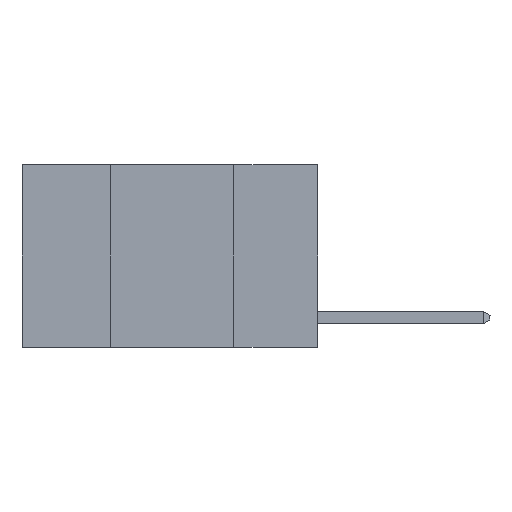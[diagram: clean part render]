
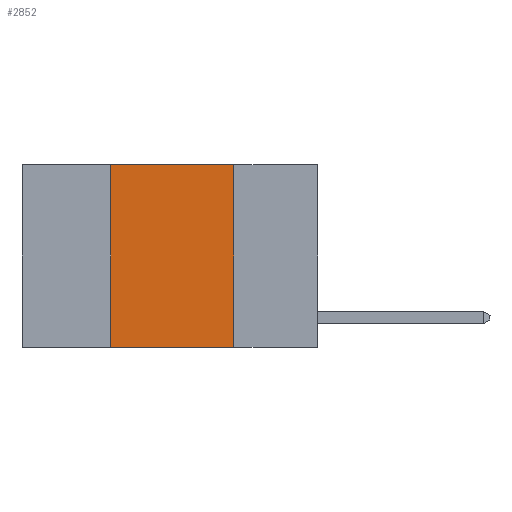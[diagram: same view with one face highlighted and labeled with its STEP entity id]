
A CAD part, left-side view. The second image highlights one B-rep face of the part: STEP entity #2852.
In plain terms, the highlighted planar face has unit normal (-1, 0, 0).
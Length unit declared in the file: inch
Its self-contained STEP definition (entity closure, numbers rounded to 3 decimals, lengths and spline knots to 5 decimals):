
#389 = CARTESIAN_POINT ( 'NONE',  ( 0., 0.42, 0. ) ) ;
#398 = DIRECTION ( 'NONE',  ( 0., -1., 0. ) ) ;
#1390 = VERTEX_POINT ( 'NONE', #5382 ) ;
#2214 = VERTEX_POINT ( 'NONE', #13376 ) ;
#2626 = EDGE_CURVE ( 'NONE', #2214, #1390, #2930, .T. ) ;
#2852 = ADVANCED_FACE ( 'NONE', ( #9622 ), #25885, .F. ) ;
#2920 = DIRECTION ( 'NONE',  ( 0., -1., 0. ) ) ;
#2930 = LINE ( 'NONE', #18603, #17862 ) ;
#4435 = EDGE_CURVE ( 'NONE', #23486, #2214, #18718, .T. ) ;
#4903 = CARTESIAN_POINT ( 'NONE',  ( 0., 0.17, -0.37 ) ) ;
#5269 = ORIENTED_EDGE ( 'NONE', *, *, #13806, .F. ) ;
#5382 = CARTESIAN_POINT ( 'NONE',  ( 0., 0.17, 0. ) ) ;
#5502 = CARTESIAN_POINT ( 'NONE',  ( 0., 0.17, 0. ) ) ;
#5900 = ORIENTED_EDGE ( 'NONE', *, *, #16000, .T. ) ;
#6391 = DIRECTION ( 'NONE',  ( 0., 0., 1. ) ) ;
#8161 = AXIS2_PLACEMENT_3D ( 'NONE', #20822, #20690, #14810 ) ;
#9157 = LINE ( 'NONE', #5502, #20582 ) ;
#9622 = FACE_OUTER_BOUND ( 'NONE', #26397, .T. ) ;
#10479 = CARTESIAN_POINT ( 'NONE',  ( 0., 0.42, -0.37 ) ) ;
#11512 = ORIENTED_EDGE ( 'NONE', *, *, #2626, .F. ) ;
#11605 = VECTOR ( 'NONE', #2920, 39.37008 ) ;
#13376 = CARTESIAN_POINT ( 'NONE',  ( 0., 0.42, 0. ) ) ;
#13806 = EDGE_CURVE ( 'NONE', #1390, #14778, #9157, .T. ) ;
#13848 = ORIENTED_EDGE ( 'NONE', *, *, #4435, .F. ) ;
#14778 = VERTEX_POINT ( 'NONE', #4903 ) ;
#14810 = DIRECTION ( 'NONE',  ( 0., 0., -1. ) ) ;
#16000 = EDGE_CURVE ( 'NONE', #23486, #14778, #22731, .T. ) ;
#17862 = VECTOR ( 'NONE', #398, 39.37008 ) ;
#18603 = CARTESIAN_POINT ( 'NONE',  ( 0., 0.6, 0. ) ) ;
#18718 = LINE ( 'NONE', #389, #19380 ) ;
#19380 = VECTOR ( 'NONE', #6391, 39.37008 ) ;
#20582 = VECTOR ( 'NONE', #21768, 39.37008 ) ;
#20690 = DIRECTION ( 'NONE',  ( 1., 0., 0. ) ) ;
#20822 = CARTESIAN_POINT ( 'NONE',  ( 0., 0.6, 0. ) ) ;
#21443 = CARTESIAN_POINT ( 'NONE',  ( 0., 0.6, -0.37 ) ) ;
#21768 = DIRECTION ( 'NONE',  ( 0., 0., -1. ) ) ;
#22731 = LINE ( 'NONE', #21443, #11605 ) ;
#23486 = VERTEX_POINT ( 'NONE', #10479 ) ;
#25885 = PLANE ( 'NONE',  #8161 ) ;
#26397 = EDGE_LOOP ( 'NONE', ( #5269, #11512, #13848, #5900 ) ) ;
